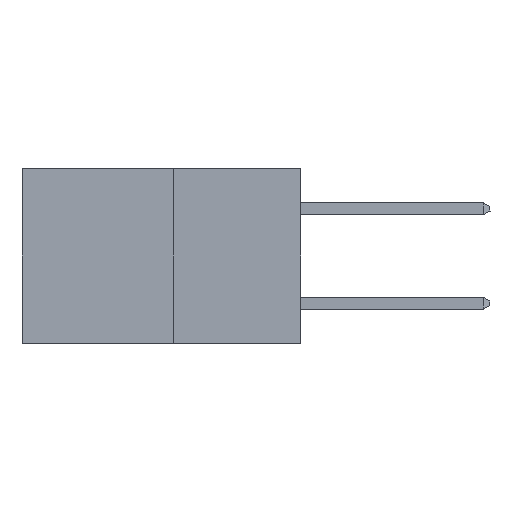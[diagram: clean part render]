
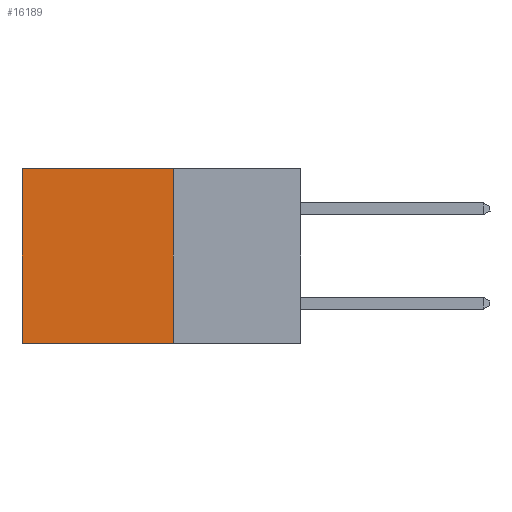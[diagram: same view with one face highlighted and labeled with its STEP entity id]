
A CAD part, left-side view. The second image highlights one B-rep face of the part: STEP entity #16189.
In plain terms, the highlighted planar face has unit normal (-1, 0, 0).
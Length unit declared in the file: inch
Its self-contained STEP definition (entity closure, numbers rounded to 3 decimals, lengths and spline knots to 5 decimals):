
#375 = VECTOR ( 'NONE', #2677, 39.37008 ) ;
#781 = CARTESIAN_POINT ( 'NONE',  ( 0.277, 0.27, 0. ) ) ;
#889 = FACE_OUTER_BOUND ( 'NONE', #16158, .T. ) ;
#966 = VECTOR ( 'NONE', #12067, 39.37008 ) ;
#1066 = VERTEX_POINT ( 'NONE', #16562 ) ;
#1205 = VERTEX_POINT ( 'NONE', #10256 ) ;
#2677 = DIRECTION ( 'NONE',  ( 0., 0., -1. ) ) ;
#3625 = VECTOR ( 'NONE', #9747, 39.37008 ) ;
#4196 = CARTESIAN_POINT ( 'NONE',  ( 0.277, 0.59, -0.37 ) ) ;
#4565 = ORIENTED_EDGE ( 'NONE', *, *, #15735, .F. ) ;
#5335 = CARTESIAN_POINT ( 'NONE',  ( 0.277, 0.27, -0.37 ) ) ;
#5974 = CARTESIAN_POINT ( 'NONE',  ( 0.277, 0.27, -0.37 ) ) ;
#6192 = DIRECTION ( 'NONE',  ( 0., 0., -1. ) ) ;
#6350 = VERTEX_POINT ( 'NONE', #6862 ) ;
#6862 = CARTESIAN_POINT ( 'NONE',  ( 0.277, 0.27, -0.37 ) ) ;
#6929 = DIRECTION ( 'NONE',  ( 1., 0., 0. ) ) ;
#7910 = LINE ( 'NONE', #10324, #3625 ) ;
#7944 = ORIENTED_EDGE ( 'NONE', *, *, #8214, .T. ) ;
#8214 = EDGE_CURVE ( 'NONE', #1066, #1205, #18490, .T. ) ;
#9747 = DIRECTION ( 'NONE',  ( 0., 1., 0. ) ) ;
#10256 = CARTESIAN_POINT ( 'NONE',  ( 0.277, 0.59, -0.37 ) ) ;
#10324 = CARTESIAN_POINT ( 'NONE',  ( 0.277, 0.27, -0.37 ) ) ;
#11013 = LINE ( 'NONE', #12173, #966 ) ;
#12067 = DIRECTION ( 'NONE',  ( 0., 1., 0. ) ) ;
#12173 = CARTESIAN_POINT ( 'NONE',  ( 0.277, 0.27, 0. ) ) ;
#12200 = AXIS2_PLACEMENT_3D ( 'NONE', #5335, #6929, #17690 ) ;
#13457 = EDGE_CURVE ( 'NONE', #6350, #1205, #7910, .T. ) ;
#13689 = VERTEX_POINT ( 'NONE', #781 ) ;
#14041 = ORIENTED_EDGE ( 'NONE', *, *, #13457, .F. ) ;
#14398 = ORIENTED_EDGE ( 'NONE', *, *, #14418, .T. ) ;
#14418 = EDGE_CURVE ( 'NONE', #13689, #1066, #11013, .T. ) ;
#15735 = EDGE_CURVE ( 'NONE', #13689, #6350, #17166, .T. ) ;
#16158 = EDGE_LOOP ( 'NONE', ( #7944, #14041, #4565, #14398 ) ) ;
#16189 = ADVANCED_FACE ( 'NONE', ( #889 ), #16210, .F. ) ;
#16210 = PLANE ( 'NONE',  #12200 ) ;
#16562 = CARTESIAN_POINT ( 'NONE',  ( 0.277, 0.59, 0. ) ) ;
#17166 = LINE ( 'NONE', #5974, #375 ) ;
#17690 = DIRECTION ( 'NONE',  ( 0., 0., -1. ) ) ;
#18048 = VECTOR ( 'NONE', #6192, 39.37008 ) ;
#18490 = LINE ( 'NONE', #4196, #18048 ) ;
